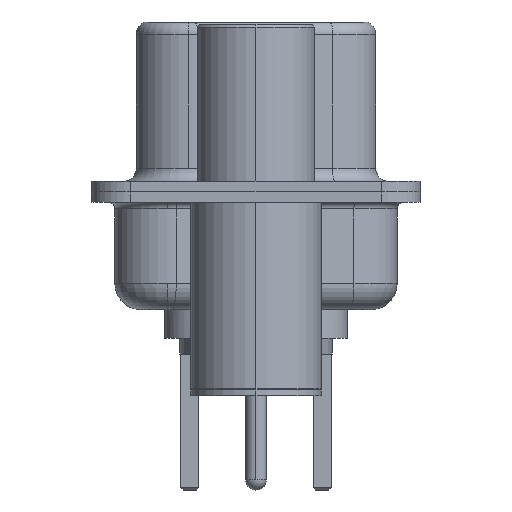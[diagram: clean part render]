
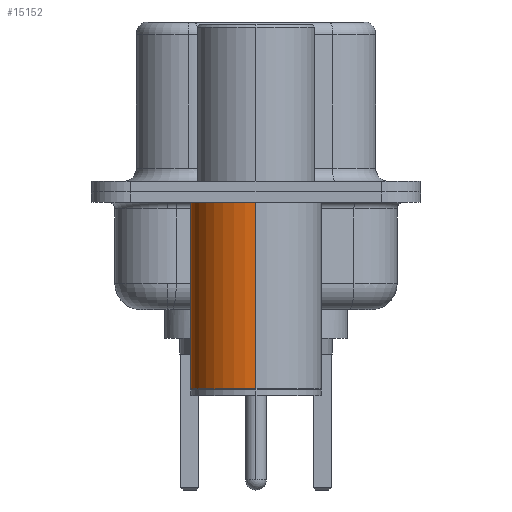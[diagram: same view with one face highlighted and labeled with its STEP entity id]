
A CAD part, left-side view. The second image highlights one B-rep face of the part: STEP entity #15152.
In plain terms, the highlighted cylindrical face has radius 2.5 mm (diameter 5 mm), a partial arc.
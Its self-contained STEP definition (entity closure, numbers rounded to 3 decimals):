
#713 = VERTEX_POINT ( 'NONE', #12471 ) ;
#1856 = CIRCLE ( 'NONE', #3114, 2.5 ) ;
#1875 = DIRECTION ( 'NONE',  ( 0., 0., 1. ) ) ;
#2385 = AXIS2_PLACEMENT_3D ( 'NONE', #13011, #1875, #14989 ) ;
#2581 = ORIENTED_EDGE ( 'NONE', *, *, #22934, .T. ) ;
#2917 = CIRCLE ( 'NONE', #2385, 2.5 ) ;
#3114 = AXIS2_PLACEMENT_3D ( 'NONE', #13100, #6386, #13878 ) ;
#3408 = EDGE_CURVE ( 'NONE', #18563, #18610, #1856, .T. ) ;
#4320 = EDGE_LOOP ( 'NONE', ( #2581, #10904, #10192, #16982 ) ) ;
#6135 = LINE ( 'NONE', #23803, #11085 ) ;
#6170 = EDGE_CURVE ( 'NONE', #713, #18563, #6135, .T. ) ;
#6386 = DIRECTION ( 'NONE',  ( 0., 0., 1. ) ) ;
#8133 = DIRECTION ( 'NONE',  ( 0., 0., 1. ) ) ;
#8220 = DIRECTION ( 'NONE',  ( 1., 0., 0. ) ) ;
#8570 = VERTEX_POINT ( 'NONE', #14695 ) ;
#8705 = CARTESIAN_POINT ( 'NONE',  ( -2.5, 0., -0.4 ) ) ;
#8911 = CARTESIAN_POINT ( 'NONE',  ( 2.5, 0., -0.4 ) ) ;
#8948 = CYLINDRICAL_SURFACE ( 'NONE', #15964, 2.5 ) ;
#10192 = ORIENTED_EDGE ( 'NONE', *, *, #3408, .F. ) ;
#10904 = ORIENTED_EDGE ( 'NONE', *, *, #17501, .T. ) ;
#11085 = VECTOR ( 'NONE', #17819, 1000. ) ;
#12471 = CARTESIAN_POINT ( 'NONE',  ( 2.5, 0., -7.525 ) ) ;
#12626 = VECTOR ( 'NONE', #17101, 1000. ) ;
#13011 = CARTESIAN_POINT ( 'NONE',  ( 0., 0., -7.525 ) ) ;
#13100 = CARTESIAN_POINT ( 'NONE',  ( 0., 0., -0.4 ) ) ;
#13878 = DIRECTION ( 'NONE',  ( 1., 0., 0. ) ) ;
#14695 = CARTESIAN_POINT ( 'NONE',  ( -2.5, 0., -7.525 ) ) ;
#14989 = DIRECTION ( 'NONE',  ( 1., 0., 0. ) ) ;
#15152 = ADVANCED_FACE ( 'NONE', ( #19384 ), #8948, .T. ) ;
#15964 = AXIS2_PLACEMENT_3D ( 'NONE', #19348, #8133, #8220 ) ;
#16982 = ORIENTED_EDGE ( 'NONE', *, *, #6170, .F. ) ;
#17101 = DIRECTION ( 'NONE',  ( 0., 0., 1. ) ) ;
#17501 = EDGE_CURVE ( 'NONE', #8570, #18610, #22397, .T. ) ;
#17819 = DIRECTION ( 'NONE',  ( 0., 0., 1. ) ) ;
#18563 = VERTEX_POINT ( 'NONE', #8911 ) ;
#18610 = VERTEX_POINT ( 'NONE', #8705 ) ;
#19348 = CARTESIAN_POINT ( 'NONE',  ( 0., 0., 0.581 ) ) ;
#19384 = FACE_OUTER_BOUND ( 'NONE', #4320, .T. ) ;
#20731 = CARTESIAN_POINT ( 'NONE',  ( -2.5, 0., 0.581 ) ) ;
#22397 = LINE ( 'NONE', #20731, #12626 ) ;
#22934 = EDGE_CURVE ( 'NONE', #713, #8570, #2917, .T. ) ;
#23803 = CARTESIAN_POINT ( 'NONE',  ( 2.5, 0., 0.581 ) ) ;
